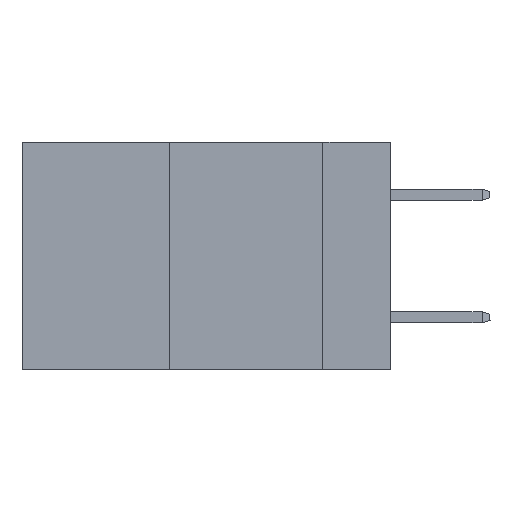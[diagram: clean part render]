
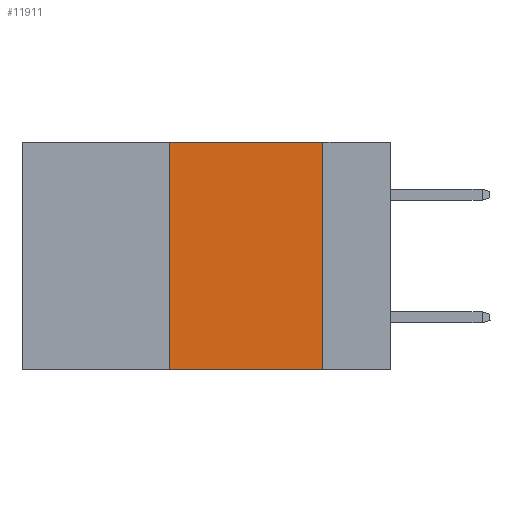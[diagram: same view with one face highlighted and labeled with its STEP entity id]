
A CAD part, left-side view. The second image highlights one B-rep face of the part: STEP entity #11911.
In plain terms, the highlighted planar face has unit normal (-1, 0, 0).
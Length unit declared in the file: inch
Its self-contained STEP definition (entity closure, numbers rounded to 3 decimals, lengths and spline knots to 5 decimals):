
#1467 = DIRECTION ( 'NONE',  ( 0., 0., -1. ) ) ;
#1473 = CARTESIAN_POINT ( 'NONE',  ( 0., 0.36, -0.37 ) ) ;
#1757 = DIRECTION ( 'NONE',  ( 0., -1., 0. ) ) ;
#1970 = CARTESIAN_POINT ( 'NONE',  ( 0., 0.11, -0.37 ) ) ;
#2888 = LINE ( 'NONE', #3070, #7349 ) ;
#3070 = CARTESIAN_POINT ( 'NONE',  ( 0., 0.6, -0.37 ) ) ;
#3377 = ORIENTED_EDGE ( 'NONE', *, *, #6612, .F. ) ;
#5771 = EDGE_CURVE ( 'NONE', #14799, #13030, #2888, .T. ) ;
#6576 = CARTESIAN_POINT ( 'NONE',  ( 0., 0.36, 0. ) ) ;
#6612 = EDGE_CURVE ( 'NONE', #14799, #16314, #13728, .T. ) ;
#6872 = AXIS2_PLACEMENT_3D ( 'NONE', #11030, #18577, #8294 ) ;
#7034 = VECTOR ( 'NONE', #11015, 39.37008 ) ;
#7038 = CARTESIAN_POINT ( 'NONE',  ( 0., 0.11, 0. ) ) ;
#7202 = DIRECTION ( 'NONE',  ( 0., -1., 0. ) ) ;
#7349 = VECTOR ( 'NONE', #1757, 39.37008 ) ;
#8094 = VECTOR ( 'NONE', #7202, 39.37008 ) ;
#8294 = DIRECTION ( 'NONE',  ( 0., 0., -1. ) ) ;
#8454 = EDGE_CURVE ( 'NONE', #10204, #13030, #8725, .T. ) ;
#8725 = LINE ( 'NONE', #7038, #16725 ) ;
#10138 = LINE ( 'NONE', #11443, #8094 ) ;
#10204 = VERTEX_POINT ( 'NONE', #18431 ) ;
#11006 = EDGE_LOOP ( 'NONE', ( #16841, #14735, #3377, #18536 ) ) ;
#11015 = DIRECTION ( 'NONE',  ( 0., 0., 1. ) ) ;
#11030 = CARTESIAN_POINT ( 'NONE',  ( 0., 0.6, 0. ) ) ;
#11443 = CARTESIAN_POINT ( 'NONE',  ( 0., 0.6, 0. ) ) ;
#11911 = ADVANCED_FACE ( 'NONE', ( #15626 ), #12804, .F. ) ;
#12804 = PLANE ( 'NONE',  #6872 ) ;
#13030 = VERTEX_POINT ( 'NONE', #1970 ) ;
#13728 = LINE ( 'NONE', #6576, #7034 ) ;
#14113 = EDGE_CURVE ( 'NONE', #16314, #10204, #10138, .T. ) ;
#14735 = ORIENTED_EDGE ( 'NONE', *, *, #14113, .F. ) ;
#14799 = VERTEX_POINT ( 'NONE', #1473 ) ;
#15626 = FACE_OUTER_BOUND ( 'NONE', #11006, .T. ) ;
#16314 = VERTEX_POINT ( 'NONE', #16642 ) ;
#16642 = CARTESIAN_POINT ( 'NONE',  ( 0., 0.36, 0. ) ) ;
#16725 = VECTOR ( 'NONE', #1467, 39.37008 ) ;
#16841 = ORIENTED_EDGE ( 'NONE', *, *, #8454, .F. ) ;
#18431 = CARTESIAN_POINT ( 'NONE',  ( 0., 0.11, 0. ) ) ;
#18536 = ORIENTED_EDGE ( 'NONE', *, *, #5771, .T. ) ;
#18577 = DIRECTION ( 'NONE',  ( 1., 0., 0. ) ) ;
